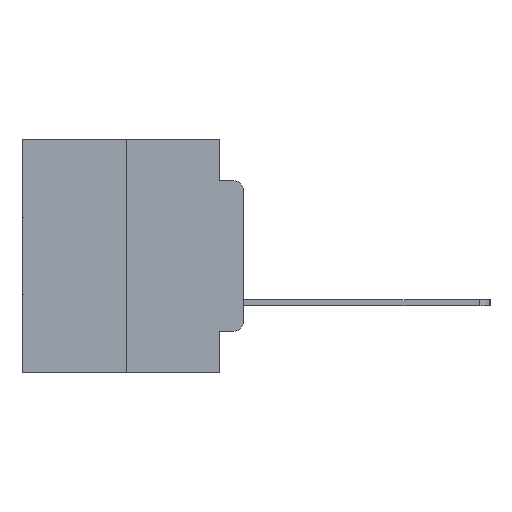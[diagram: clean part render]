
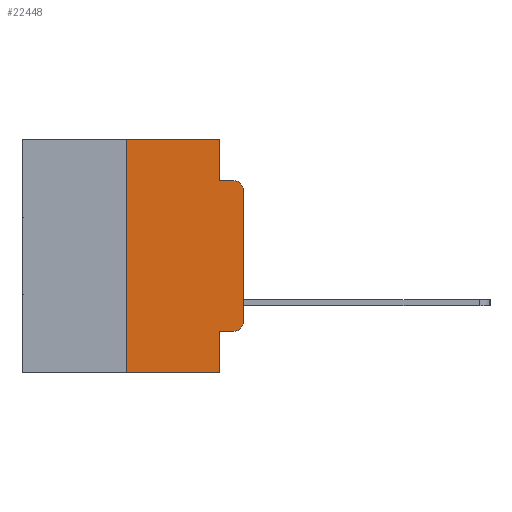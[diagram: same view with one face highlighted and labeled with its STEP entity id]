
A CAD part, left-side view. The second image highlights one B-rep face of the part: STEP entity #22448.
In plain terms, the highlighted planar face has unit normal (-1, 0, 0).
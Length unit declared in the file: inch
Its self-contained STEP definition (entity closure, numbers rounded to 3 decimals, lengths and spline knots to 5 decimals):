
#333 = DIRECTION ( 'NONE',  ( 0., 0., 1. ) ) ;
#629 = ORIENTED_EDGE ( 'NONE', *, *, #21795, .T. ) ;
#850 = VERTEX_POINT ( 'NONE', #25830 ) ;
#1738 = LINE ( 'NONE', #10107, #23515 ) ;
#1943 = VERTEX_POINT ( 'NONE', #6552 ) ;
#2039 = DIRECTION ( 'NONE',  ( 0., -1., 0. ) ) ;
#2317 = CARTESIAN_POINT ( 'NONE',  ( 0., 0., -0.3915 ) ) ;
#2648 = CIRCLE ( 'NONE', #25817, 0.02 ) ;
#2692 = EDGE_CURVE ( 'NONE', #14906, #25545, #6376, .T. ) ;
#2992 = CARTESIAN_POINT ( 'NONE',  ( 0., 0.051, -0.5 ) ) ;
#3279 = CARTESIAN_POINT ( 'NONE',  ( 0., 0.051, -0.4115 ) ) ;
#3855 = LINE ( 'NONE', #11766, #20099 ) ;
#4088 = CARTESIAN_POINT ( 'NONE',  ( 0., 0.02, -0.1085 ) ) ;
#4155 = DIRECTION ( 'NONE',  ( 1., 0., 0. ) ) ;
#4293 = CARTESIAN_POINT ( 'NONE',  ( 0., 0.473, -0.5 ) ) ;
#5189 = VECTOR ( 'NONE', #24099, 39.37008 ) ;
#5953 = DIRECTION ( 'NONE',  ( -1., 0., 0. ) ) ;
#6058 = DIRECTION ( 'NONE',  ( 0., 0., -1. ) ) ;
#6242 = DIRECTION ( 'NONE',  ( 0., 0., -1. ) ) ;
#6376 = LINE ( 'NONE', #4293, #15696 ) ;
#6552 = CARTESIAN_POINT ( 'NONE',  ( 0., 0.051, -0.0885 ) ) ;
#7145 = CARTESIAN_POINT ( 'NONE',  ( 0., 0.25, -0.5 ) ) ;
#7439 = ORIENTED_EDGE ( 'NONE', *, *, #12854, .F. ) ;
#7923 = CARTESIAN_POINT ( 'NONE',  ( 0., 0., -0.1085 ) ) ;
#8303 = CARTESIAN_POINT ( 'NONE',  ( 0., 0.473, 0. ) ) ;
#8637 = EDGE_CURVE ( 'NONE', #14906, #13399, #3855, .T. ) ;
#9097 = LINE ( 'NONE', #16679, #9761 ) ;
#9519 = CARTESIAN_POINT ( 'NONE',  ( 0., 0.473, 0. ) ) ;
#9600 = CARTESIAN_POINT ( 'NONE',  ( 0., 0.02, -0.0885 ) ) ;
#9761 = VECTOR ( 'NONE', #6058, 39.37008 ) ;
#10107 = CARTESIAN_POINT ( 'NONE',  ( 0., 0.051, 0. ) ) ;
#11452 = EDGE_CURVE ( 'NONE', #11468, #1943, #1738, .T. ) ;
#11468 = VERTEX_POINT ( 'NONE', #12215 ) ;
#11702 = LINE ( 'NONE', #18988, #16688 ) ;
#11766 = CARTESIAN_POINT ( 'NONE',  ( 0., 0.25, 0. ) ) ;
#12215 = CARTESIAN_POINT ( 'NONE',  ( 0., 0.051, 0. ) ) ;
#12854 = EDGE_CURVE ( 'NONE', #1943, #26955, #11702, .T. ) ;
#12856 = FACE_OUTER_BOUND ( 'NONE', #15874, .T. ) ;
#12862 = VECTOR ( 'NONE', #2039, 39.37008 ) ;
#13069 = ORIENTED_EDGE ( 'NONE', *, *, #11452, .F. ) ;
#13195 = VERTEX_POINT ( 'NONE', #3279 ) ;
#13393 = ORIENTED_EDGE ( 'NONE', *, *, #2692, .T. ) ;
#13399 = VERTEX_POINT ( 'NONE', #18861 ) ;
#14408 = ORIENTED_EDGE ( 'NONE', *, *, #19923, .T. ) ;
#14843 = CARTESIAN_POINT ( 'NONE',  ( 0., 0.051, -0.4115 ) ) ;
#14906 = VERTEX_POINT ( 'NONE', #7145 ) ;
#15696 = VECTOR ( 'NONE', #18052, 39.37008 ) ;
#15714 = EDGE_CURVE ( 'NONE', #27069, #26955, #19181, .T. ) ;
#15874 = EDGE_LOOP ( 'NONE', ( #14408, #25389, #7439, #13069, #25689, #27003, #13393, #20313, #19973, #629 ) ) ;
#16095 = VECTOR ( 'NONE', #333, 39.37008 ) ;
#16679 = CARTESIAN_POINT ( 'NONE',  ( 0., 0.051, 0. ) ) ;
#16688 = VECTOR ( 'NONE', #23095, 39.37008 ) ;
#17687 = EDGE_CURVE ( 'NONE', #13399, #11468, #21377, .T. ) ;
#18052 = DIRECTION ( 'NONE',  ( 0., -1., 0. ) ) ;
#18483 = LINE ( 'NONE', #14843, #12862 ) ;
#18647 = CARTESIAN_POINT ( 'NONE',  ( 0., 0.02, -0.3915 ) ) ;
#18861 = CARTESIAN_POINT ( 'NONE',  ( 0., 0.25, 0. ) ) ;
#18904 = PLANE ( 'NONE',  #24796 ) ;
#18931 = DIRECTION ( 'NONE',  ( -1., 0., 0. ) ) ;
#18988 = CARTESIAN_POINT ( 'NONE',  ( 0., 0.051, -0.0885 ) ) ;
#18997 = DIRECTION ( 'NONE',  ( 0., 0., -1. ) ) ;
#19181 = CIRCLE ( 'NONE', #25900, 0.02 ) ;
#19923 = EDGE_CURVE ( 'NONE', #21302, #27069, #21610, .T. ) ;
#19973 = ORIENTED_EDGE ( 'NONE', *, *, #23144, .T. ) ;
#20099 = VECTOR ( 'NONE', #22172, 39.37008 ) ;
#20313 = ORIENTED_EDGE ( 'NONE', *, *, #25873, .F. ) ;
#20747 = DIRECTION ( 'NONE',  ( 0., 0., -1. ) ) ;
#21302 = VERTEX_POINT ( 'NONE', #2317 ) ;
#21377 = LINE ( 'NONE', #9519, #5189 ) ;
#21610 = LINE ( 'NONE', #23582, #16095 ) ;
#21795 = EDGE_CURVE ( 'NONE', #850, #21302, #2648, .T. ) ;
#22172 = DIRECTION ( 'NONE',  ( 0., 0., 1. ) ) ;
#22448 = ADVANCED_FACE ( 'NONE', ( #12856 ), #18904, .F. ) ;
#23095 = DIRECTION ( 'NONE',  ( 0., -1., 0. ) ) ;
#23144 = EDGE_CURVE ( 'NONE', #13195, #850, #18483, .T. ) ;
#23515 = VECTOR ( 'NONE', #26715, 39.37008 ) ;
#23582 = CARTESIAN_POINT ( 'NONE',  ( 0., 0., 0. ) ) ;
#24099 = DIRECTION ( 'NONE',  ( 0., -1., 0. ) ) ;
#24796 = AXIS2_PLACEMENT_3D ( 'NONE', #8303, #4155, #18997 ) ;
#25389 = ORIENTED_EDGE ( 'NONE', *, *, #15714, .T. ) ;
#25545 = VERTEX_POINT ( 'NONE', #2992 ) ;
#25689 = ORIENTED_EDGE ( 'NONE', *, *, #17687, .F. ) ;
#25817 = AXIS2_PLACEMENT_3D ( 'NONE', #18647, #5953, #20747 ) ;
#25830 = CARTESIAN_POINT ( 'NONE',  ( 0., 0.02, -0.4115 ) ) ;
#25873 = EDGE_CURVE ( 'NONE', #13195, #25545, #9097, .T. ) ;
#25900 = AXIS2_PLACEMENT_3D ( 'NONE', #4088, #18931, #6242 ) ;
#26715 = DIRECTION ( 'NONE',  ( 0., 0., -1. ) ) ;
#26955 = VERTEX_POINT ( 'NONE', #9600 ) ;
#27003 = ORIENTED_EDGE ( 'NONE', *, *, #8637, .F. ) ;
#27069 = VERTEX_POINT ( 'NONE', #7923 ) ;
